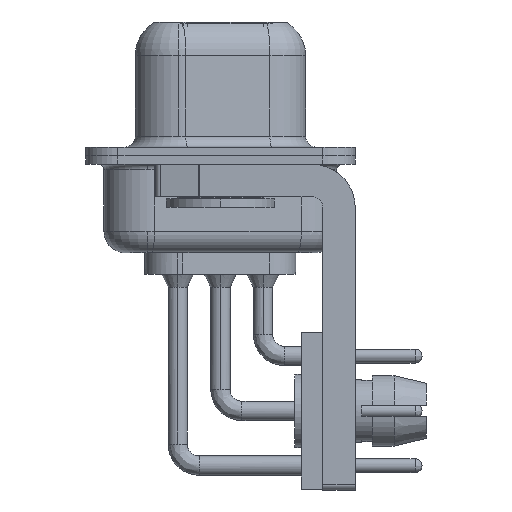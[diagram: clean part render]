
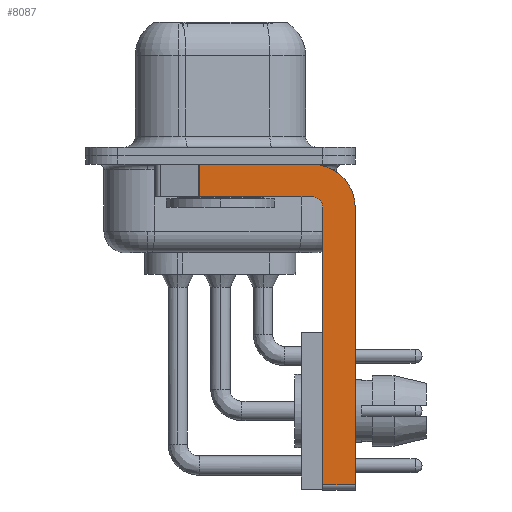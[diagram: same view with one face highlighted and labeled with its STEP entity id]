
A CAD part, left-side view. The second image highlights one B-rep face of the part: STEP entity #8087.
In plain terms, the highlighted planar face has unit normal (-1, 0, 0).
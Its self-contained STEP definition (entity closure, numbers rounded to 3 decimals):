
#161 = EDGE_CURVE ( 'NONE', #14171, #7309, #6534, .T. ) ;
#509 = CARTESIAN_POINT ( 'NONE',  ( -2.9, -4.75, -15.25 ) ) ;
#896 = EDGE_CURVE ( 'NONE', #8485, #24243, #16241, .T. ) ;
#1793 = CARTESIAN_POINT ( 'NONE',  ( -2.9, -4.25, -0.4 ) ) ;
#1931 = CARTESIAN_POINT ( 'NONE',  ( -2.9, -6.25, -15.25 ) ) ;
#3696 = ORIENTED_EDGE ( 'NONE', *, *, #21566, .F. ) ;
#3909 = VERTEX_POINT ( 'NONE', #1931 ) ;
#5049 = AXIS2_PLACEMENT_3D ( 'NONE', #24253, #7264, #27101 ) ;
#5189 = DIRECTION ( 'NONE',  ( 1., 0., 0. ) ) ;
#5230 = CARTESIAN_POINT ( 'NONE',  ( -2.9, -4.75, -2.4 ) ) ;
#6247 = FACE_OUTER_BOUND ( 'NONE', #14999, .T. ) ;
#6534 = LINE ( 'NONE', #26242, #14043 ) ;
#7264 = DIRECTION ( 'NONE',  ( -1., 0., 0. ) ) ;
#7309 = VERTEX_POINT ( 'NONE', #30560 ) ;
#8087 = ADVANCED_FACE ( 'NONE', ( #6247 ), #10664, .F. ) ;
#8485 = VERTEX_POINT ( 'NONE', #1793 ) ;
#8810 = CARTESIAN_POINT ( 'NONE',  ( -2.9, -4.25, -15.25 ) ) ;
#10664 = PLANE ( 'NONE',  #26081 ) ;
#11219 = CARTESIAN_POINT ( 'NONE',  ( -2.9, 3., -0.4 ) ) ;
#11586 = VERTEX_POINT ( 'NONE', #5230 ) ;
#12214 = CARTESIAN_POINT ( 'NONE',  ( -2.9, -6.25, -2.4 ) ) ;
#13182 = ORIENTED_EDGE ( 'NONE', *, *, #29986, .F. ) ;
#14043 = VECTOR ( 'NONE', #32068, 1000. ) ;
#14171 = VERTEX_POINT ( 'NONE', #33155 ) ;
#14280 = ORIENTED_EDGE ( 'NONE', *, *, #32702, .F. ) ;
#14895 = ORIENTED_EDGE ( 'NONE', *, *, #896, .F. ) ;
#14999 = EDGE_LOOP ( 'NONE', ( #3696, #29933, #24029, #13182, #18113, #18513, #14280, #14895 ) ) ;
#15001 = CARTESIAN_POINT ( 'NONE',  ( -2.9, -6.25, -2.4 ) ) ;
#15066 = DIRECTION ( 'NONE',  ( 0., 0., -1. ) ) ;
#16241 = CIRCLE ( 'NONE', #23531, 2. ) ;
#18113 = ORIENTED_EDGE ( 'NONE', *, *, #34146, .F. ) ;
#18456 = EDGE_CURVE ( 'NONE', #29759, #3909, #33941, .T. ) ;
#18513 = ORIENTED_EDGE ( 'NONE', *, *, #18456, .T. ) ;
#18795 = DIRECTION ( 'NONE',  ( 0., 0., -1. ) ) ;
#20406 = CARTESIAN_POINT ( 'NONE',  ( -2.9, 0.978, -0.4 ) ) ;
#21566 = EDGE_CURVE ( 'NONE', #29758, #8485, #36543, .T. ) ;
#22041 = CARTESIAN_POINT ( 'NONE',  ( -2.9, -4.75, -15.5 ) ) ;
#22720 = CARTESIAN_POINT ( 'NONE',  ( -2.9, -4.25, -2.4 ) ) ;
#23388 = LINE ( 'NONE', #12214, #36826 ) ;
#23531 = AXIS2_PLACEMENT_3D ( 'NONE', #22720, #28217, #28333 ) ;
#24029 = ORIENTED_EDGE ( 'NONE', *, *, #161, .F. ) ;
#24047 = CIRCLE ( 'NONE', #5049, 0.5 ) ;
#24243 = VERTEX_POINT ( 'NONE', #15001 ) ;
#24253 = CARTESIAN_POINT ( 'NONE',  ( -2.9, -4.25, -2.4 ) ) ;
#24899 = EDGE_CURVE ( 'NONE', #29758, #7309, #35041, .T. ) ;
#25075 = DIRECTION ( 'NONE',  ( 0., 0., -1. ) ) ;
#25967 = VECTOR ( 'NONE', #30670, 1000. ) ;
#26081 = AXIS2_PLACEMENT_3D ( 'NONE', #36490, #5189, #25075 ) ;
#26242 = CARTESIAN_POINT ( 'NONE',  ( -2.9, -4.25, -1.9 ) ) ;
#26286 = VECTOR ( 'NONE', #34359, 1000. ) ;
#27085 = VECTOR ( 'NONE', #36790, 1000. ) ;
#27101 = DIRECTION ( 'NONE',  ( 0., 0., 1. ) ) ;
#27385 = VECTOR ( 'NONE', #18795, 1000. ) ;
#28217 = DIRECTION ( 'NONE',  ( 1., 0., 0. ) ) ;
#28333 = DIRECTION ( 'NONE',  ( 0., 0., -1. ) ) ;
#29758 = VERTEX_POINT ( 'NONE', #20406 ) ;
#29759 = VERTEX_POINT ( 'NONE', #509 ) ;
#29933 = ORIENTED_EDGE ( 'NONE', *, *, #24899, .T. ) ;
#29986 = EDGE_CURVE ( 'NONE', #11586, #14171, #24047, .T. ) ;
#30560 = CARTESIAN_POINT ( 'NONE',  ( -2.9, 0.978, -1.9 ) ) ;
#30670 = DIRECTION ( 'NONE',  ( 0., 0., 1. ) ) ;
#32068 = DIRECTION ( 'NONE',  ( 0., 1., 0. ) ) ;
#32702 = EDGE_CURVE ( 'NONE', #24243, #3909, #23388, .T. ) ;
#33064 = CARTESIAN_POINT ( 'NONE',  ( -2.9, 0.978, -1.9 ) ) ;
#33155 = CARTESIAN_POINT ( 'NONE',  ( -2.9, -4.25, -1.9 ) ) ;
#33630 = LINE ( 'NONE', #22041, #25967 ) ;
#33941 = LINE ( 'NONE', #8810, #26286 ) ;
#34146 = EDGE_CURVE ( 'NONE', #29759, #11586, #33630, .T. ) ;
#34359 = DIRECTION ( 'NONE',  ( 0., -1., 0. ) ) ;
#35041 = LINE ( 'NONE', #33064, #27385 ) ;
#36490 = CARTESIAN_POINT ( 'NONE',  ( -2.9, -4.25, -2.4 ) ) ;
#36543 = LINE ( 'NONE', #11219, #27085 ) ;
#36790 = DIRECTION ( 'NONE',  ( 0., -1., 0. ) ) ;
#36826 = VECTOR ( 'NONE', #15066, 1000. ) ;
